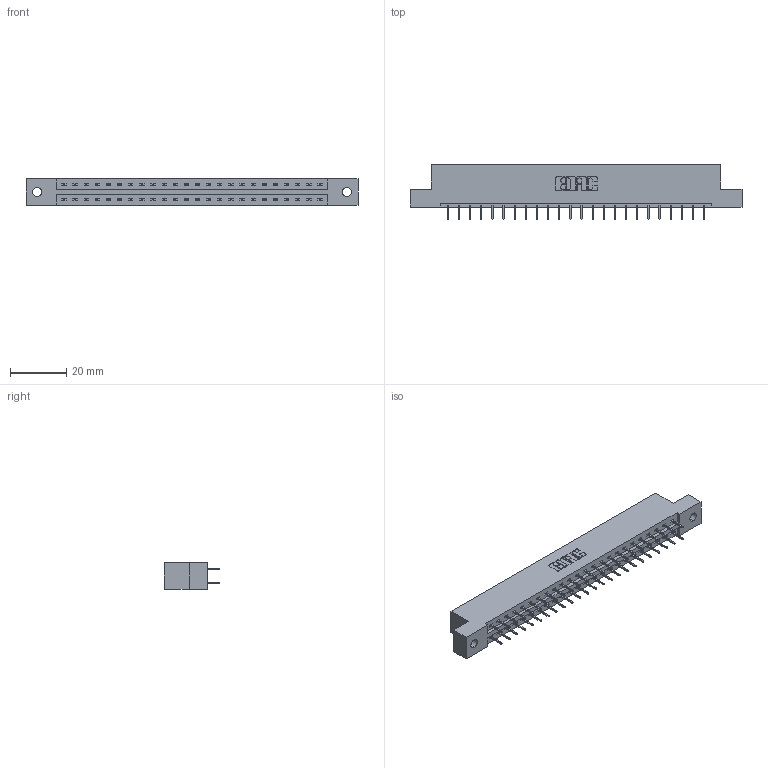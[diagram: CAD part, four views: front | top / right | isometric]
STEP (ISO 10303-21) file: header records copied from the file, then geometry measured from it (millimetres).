
FILE_DESCRIPTION (( 'STEP AP203' ), '1' );
FILE_NAME ('387-048-524-202.STEP', '2018-09-20T05:39:14', ( '' ), ( '' ), 'SwSTEP 2.0', 'SolidWorks 2016', '' );
FILE_SCHEMA (( 'CONFIG_CONTROL_DESIGN' ));
Length unit declared in the file: inch
Products named in the file (3): 345-292-001_345-293-124; 387-048-524-202; 337 Part_Flush Mounting Lugs - 0.128 Dia
Assembly tree (49 placements, depth 2):
  387-048-524-202
    337 Part_Flush Mounting Lugs - 0.128 Dia
    345-292-001_345-293-124  x48
Bounding box: 118.11 x 19.69 x 9.4 mm (x, y, z)
Volume: 12098.4 mm3; surface area: 13004.8 mm2
Topology: 49 solids, 49 shells, 2898 faces, 8231 edges, 5294 vertices
Faces by surface type: plane 2182, cylinder 716
Entity records: 21013 total; most frequent: CARTESIAN_POINT 3554, ORIENTED_EDGE 3490, DIRECTION 3057, EDGE_CURVE 1745, VECTOR 1621, LINE 1621, VERTEX_POINT 1158, AXIS2_PLACEMENT_3D 718
